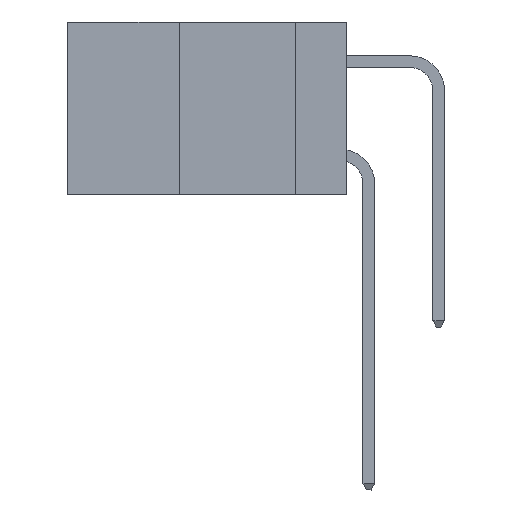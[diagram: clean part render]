
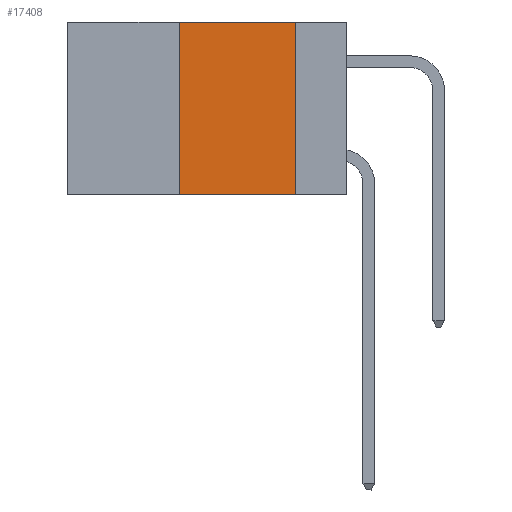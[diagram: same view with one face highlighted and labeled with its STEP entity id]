
A CAD part, left-side view. The second image highlights one B-rep face of the part: STEP entity #17408.
In plain terms, the highlighted planar face has unit normal (-1, 0, 0).
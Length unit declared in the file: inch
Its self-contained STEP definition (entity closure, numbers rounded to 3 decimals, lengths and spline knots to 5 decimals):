
#19 = EDGE_LOOP ( 'NONE', ( #1061, #13742, #2083, #18778 ) ) ;
#1061 = ORIENTED_EDGE ( 'NONE', *, *, #6768, .F. ) ;
#1359 = LINE ( 'NONE', #4427, #10653 ) ;
#1860 = DIRECTION ( 'NONE',  ( 1., 0., 0. ) ) ;
#2083 = ORIENTED_EDGE ( 'NONE', *, *, #10686, .F. ) ;
#2380 = AXIS2_PLACEMENT_3D ( 'NONE', #8946, #1860, #14786 ) ;
#3113 = CARTESIAN_POINT ( 'NONE',  ( 0., 0.11, -0.37 ) ) ;
#3544 = CARTESIAN_POINT ( 'NONE',  ( 0., 0.36, 0. ) ) ;
#3947 = VERTEX_POINT ( 'NONE', #9252 ) ;
#4427 = CARTESIAN_POINT ( 'NONE',  ( 0., 0.6, -0.37 ) ) ;
#4940 = FACE_OUTER_BOUND ( 'NONE', #19, .T. ) ;
#5981 = CARTESIAN_POINT ( 'NONE',  ( 0., 0.6, 0. ) ) ;
#6388 = VERTEX_POINT ( 'NONE', #12412 ) ;
#6449 = EDGE_CURVE ( 'NONE', #7733, #3947, #10090, .T. ) ;
#6454 = PLANE ( 'NONE',  #2380 ) ;
#6556 = DIRECTION ( 'NONE',  ( 0., 0., -1. ) ) ;
#6645 = LINE ( 'NONE', #13932, #16667 ) ;
#6768 = EDGE_CURVE ( 'NONE', #3947, #12927, #6645, .T. ) ;
#7733 = VERTEX_POINT ( 'NONE', #14324 ) ;
#7945 = LINE ( 'NONE', #3544, #13245 ) ;
#8572 = DIRECTION ( 'NONE',  ( 0., -1., 0. ) ) ;
#8829 = DIRECTION ( 'NONE',  ( 0., -1., 0. ) ) ;
#8946 = CARTESIAN_POINT ( 'NONE',  ( 0., 0.6, 0. ) ) ;
#8991 = VECTOR ( 'NONE', #8572, 39.37008 ) ;
#9252 = CARTESIAN_POINT ( 'NONE',  ( 0., 0.11, 0. ) ) ;
#10090 = LINE ( 'NONE', #5981, #8991 ) ;
#10653 = VECTOR ( 'NONE', #8829, 39.37008 ) ;
#10686 = EDGE_CURVE ( 'NONE', #6388, #7733, #7945, .T. ) ;
#12412 = CARTESIAN_POINT ( 'NONE',  ( 0., 0.36, -0.37 ) ) ;
#12927 = VERTEX_POINT ( 'NONE', #3113 ) ;
#13245 = VECTOR ( 'NONE', #13608, 39.37008 ) ;
#13608 = DIRECTION ( 'NONE',  ( 0., 0., 1. ) ) ;
#13742 = ORIENTED_EDGE ( 'NONE', *, *, #6449, .F. ) ;
#13932 = CARTESIAN_POINT ( 'NONE',  ( 0., 0.11, 0. ) ) ;
#14324 = CARTESIAN_POINT ( 'NONE',  ( 0., 0.36, 0. ) ) ;
#14786 = DIRECTION ( 'NONE',  ( 0., 0., -1. ) ) ;
#16667 = VECTOR ( 'NONE', #6556, 39.37008 ) ;
#17408 = ADVANCED_FACE ( 'NONE', ( #4940 ), #6454, .F. ) ;
#17709 = EDGE_CURVE ( 'NONE', #6388, #12927, #1359, .T. ) ;
#18778 = ORIENTED_EDGE ( 'NONE', *, *, #17709, .T. ) ;
